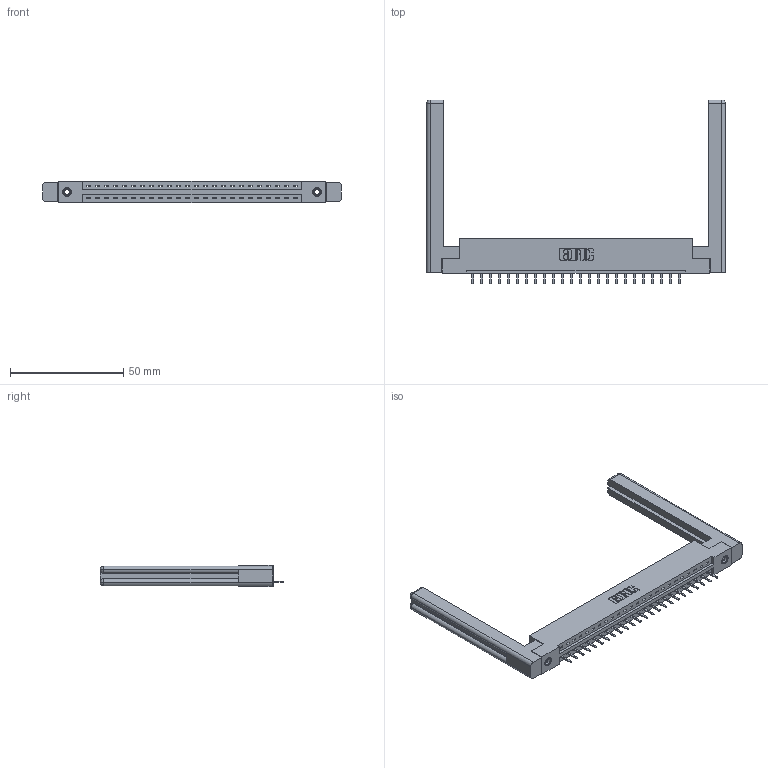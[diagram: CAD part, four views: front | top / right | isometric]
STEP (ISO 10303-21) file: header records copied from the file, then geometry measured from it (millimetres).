
FILE_DESCRIPTION (( 'STEP AP203' ), '1' );
FILE_NAME ('337-024-520-158.STEP', '2019-09-30T15:19:58', ( '' ), ( '' ), 'SwSTEP 2.0', 'SolidWorks 2016', '' );
FILE_SCHEMA (( 'CONFIG_CONTROL_DESIGN' ));
Length unit declared in the file: inch
Products named in the file (5): 307-220-058; 345-292-001_345-293-120; 337 Part_Flush Mounting Lugs - 0.156 Dia-TI; 345-250-001_345-250-001-102; 337-024-520-158
Assembly tree (29 placements, depth 2):
  337-024-520-158
    337 Part_Flush Mounting Lugs - 0.156 Dia-TI
    345-292-001_345-293-120  x24
    345-250-001_345-250-001-102  x2
    307-220-058  x2
Bounding box: 131.72 x 81.11 x 9.4 mm (x, y, z)
Volume: 20558.4 mm3; surface area: 18707.7 mm2
Topology: 29 solids, 29 shells, 1840 faces, 5369 edges, 3502 vertices
Faces by surface type: plane 1306, cylinder 510, cone 12, torus 12
Entity records: 22916 total; most frequent: CARTESIAN_POINT 4001, ORIENTED_EDGE 3888, DIRECTION 3412, EDGE_CURVE 1944, VECTOR 1764, LINE 1764, VERTEX_POINT 1286, AXIS2_PLACEMENT_3D 824
